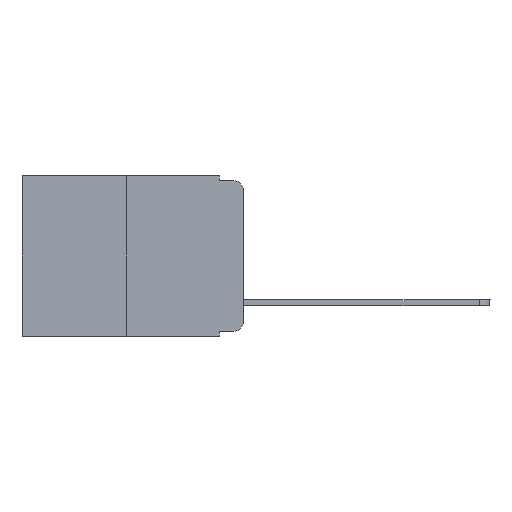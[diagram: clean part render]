
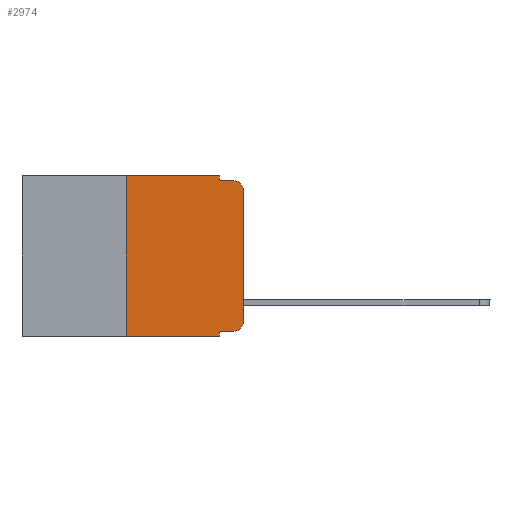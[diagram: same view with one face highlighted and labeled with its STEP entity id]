
A CAD part, left-side view. The second image highlights one B-rep face of the part: STEP entity #2974.
In plain terms, the highlighted planar face has unit normal (-1, 0, 0).
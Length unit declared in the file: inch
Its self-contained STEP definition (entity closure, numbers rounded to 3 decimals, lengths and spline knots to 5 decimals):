
#389 = LINE ( 'NONE', #3741, #22636 ) ;
#976 = CARTESIAN_POINT ( 'NONE',  ( 0., 0.25, 0. ) ) ;
#1397 = DIRECTION ( 'NONE',  ( 0., 0., 1. ) ) ;
#1466 = DIRECTION ( 'NONE',  ( 0., 0., -1. ) ) ;
#1766 = VERTEX_POINT ( 'NONE', #20906 ) ;
#1799 = EDGE_CURVE ( 'NONE', #18498, #20339, #9562, .T. ) ;
#2149 = CARTESIAN_POINT ( 'NONE',  ( 0., 0.25, -0.343 ) ) ;
#2675 = DIRECTION ( 'NONE',  ( 0., -1., 0. ) ) ;
#2742 = CARTESIAN_POINT ( 'NONE',  ( 0., 0.051, -0.333 ) ) ;
#2803 = LINE ( 'NONE', #976, #7537 ) ;
#2889 = DIRECTION ( 'NONE',  ( 0., 0., 1. ) ) ;
#2974 = ADVANCED_FACE ( 'NONE', ( #15620 ), #15904, .F. ) ;
#3198 = EDGE_CURVE ( 'NONE', #24201, #20629, #23777, .T. ) ;
#3352 = LINE ( 'NONE', #2742, #7173 ) ;
#3597 = CARTESIAN_POINT ( 'NONE',  ( 0., 0., -0.313 ) ) ;
#3741 = CARTESIAN_POINT ( 'NONE',  ( 0., 0.051, -0.01 ) ) ;
#4355 = ORIENTED_EDGE ( 'NONE', *, *, #20521, .T. ) ;
#4541 = DIRECTION ( 'NONE',  ( 0., -1., 0. ) ) ;
#4704 = CARTESIAN_POINT ( 'NONE',  ( 0., 0.473, 0. ) ) ;
#4723 = EDGE_CURVE ( 'NONE', #20629, #5110, #20516, .T. ) ;
#5110 = VERTEX_POINT ( 'NONE', #7577 ) ;
#5482 = CARTESIAN_POINT ( 'NONE',  ( 0., 0.051, 0. ) ) ;
#5910 = DIRECTION ( 'NONE',  ( 0., -1., 0. ) ) ;
#6324 = CIRCLE ( 'NONE', #9979, 0.02 ) ;
#6685 = VECTOR ( 'NONE', #2675, 39.37008 ) ;
#7173 = VECTOR ( 'NONE', #4541, 39.37008 ) ;
#7537 = VECTOR ( 'NONE', #2889, 39.37008 ) ;
#7577 = CARTESIAN_POINT ( 'NONE',  ( 0., 0.02, -0.01 ) ) ;
#7585 = VERTEX_POINT ( 'NONE', #2149 ) ;
#7666 = VERTEX_POINT ( 'NONE', #21299 ) ;
#8234 = EDGE_CURVE ( 'NONE', #7585, #7666, #18344, .T. ) ;
#8530 = ORIENTED_EDGE ( 'NONE', *, *, #14546, .F. ) ;
#8667 = EDGE_CURVE ( 'NONE', #7585, #14460, #2803, .T. ) ;
#8802 = AXIS2_PLACEMENT_3D ( 'NONE', #18492, #12857, #1466 ) ;
#9562 = LINE ( 'NONE', #9573, #13900 ) ;
#9573 = CARTESIAN_POINT ( 'NONE',  ( 0., 0.051, 0. ) ) ;
#9606 = ORIENTED_EDGE ( 'NONE', *, *, #1799, .F. ) ;
#9736 = EDGE_CURVE ( 'NONE', #14381, #1766, #3352, .T. ) ;
#9851 = ORIENTED_EDGE ( 'NONE', *, *, #4723, .T. ) ;
#9979 = AXIS2_PLACEMENT_3D ( 'NONE', #14351, #10777, #10848 ) ;
#10173 = EDGE_CURVE ( 'NONE', #14381, #7666, #13553, .T. ) ;
#10641 = VECTOR ( 'NONE', #15260, 39.37008 ) ;
#10777 = DIRECTION ( 'NONE',  ( -1., 0., 0. ) ) ;
#10848 = DIRECTION ( 'NONE',  ( 0., 0., -1. ) ) ;
#11350 = ORIENTED_EDGE ( 'NONE', *, *, #17610, .F. ) ;
#11405 = DIRECTION ( 'NONE',  ( 0., 0., -1. ) ) ;
#12857 = DIRECTION ( 'NONE',  ( -1., 0., 0. ) ) ;
#13503 = EDGE_LOOP ( 'NONE', ( #19435, #9851, #8530, #9606, #11350, #23774, #15756, #16168, #20998, #4355 ) ) ;
#13553 = LINE ( 'NONE', #5482, #10641 ) ;
#13656 = CARTESIAN_POINT ( 'NONE',  ( 0., 0.473, -0.343 ) ) ;
#13900 = VECTOR ( 'NONE', #11405, 39.37008 ) ;
#14351 = CARTESIAN_POINT ( 'NONE',  ( 0., 0.02, -0.313 ) ) ;
#14381 = VERTEX_POINT ( 'NONE', #22117 ) ;
#14460 = VERTEX_POINT ( 'NONE', #14512 ) ;
#14512 = CARTESIAN_POINT ( 'NONE',  ( 0., 0.25, 0. ) ) ;
#14543 = VECTOR ( 'NONE', #19277, 39.37008 ) ;
#14546 = EDGE_CURVE ( 'NONE', #20339, #5110, #389, .T. ) ;
#14588 = LINE ( 'NONE', #17785, #6685 ) ;
#15076 = CARTESIAN_POINT ( 'NONE',  ( 0., 0., -0.03 ) ) ;
#15260 = DIRECTION ( 'NONE',  ( 0., 0., -1. ) ) ;
#15597 = VECTOR ( 'NONE', #1397, 39.37008 ) ;
#15620 = FACE_OUTER_BOUND ( 'NONE', #13503, .T. ) ;
#15756 = ORIENTED_EDGE ( 'NONE', *, *, #8234, .T. ) ;
#15898 = CARTESIAN_POINT ( 'NONE',  ( 0., 0.051, -0.01 ) ) ;
#15904 = PLANE ( 'NONE',  #22057 ) ;
#16168 = ORIENTED_EDGE ( 'NONE', *, *, #10173, .F. ) ;
#16379 = CARTESIAN_POINT ( 'NONE',  ( 0., 0., 0. ) ) ;
#17610 = EDGE_CURVE ( 'NONE', #14460, #18498, #14588, .T. ) ;
#17776 = DIRECTION ( 'NONE',  ( 1., 0., 0. ) ) ;
#17785 = CARTESIAN_POINT ( 'NONE',  ( 0., 0.473, 0. ) ) ;
#18256 = CARTESIAN_POINT ( 'NONE',  ( 0., 0.051, 0. ) ) ;
#18344 = LINE ( 'NONE', #13656, #14543 ) ;
#18492 = CARTESIAN_POINT ( 'NONE',  ( 0., 0.02, -0.03 ) ) ;
#18498 = VERTEX_POINT ( 'NONE', #18256 ) ;
#19277 = DIRECTION ( 'NONE',  ( 0., -1., 0. ) ) ;
#19435 = ORIENTED_EDGE ( 'NONE', *, *, #3198, .T. ) ;
#19662 = DIRECTION ( 'NONE',  ( 0., 0., -1. ) ) ;
#20339 = VERTEX_POINT ( 'NONE', #15898 ) ;
#20516 = CIRCLE ( 'NONE', #8802, 0.02 ) ;
#20521 = EDGE_CURVE ( 'NONE', #1766, #24201, #6324, .T. ) ;
#20629 = VERTEX_POINT ( 'NONE', #15076 ) ;
#20906 = CARTESIAN_POINT ( 'NONE',  ( 0., 0.02, -0.333 ) ) ;
#20998 = ORIENTED_EDGE ( 'NONE', *, *, #9736, .T. ) ;
#21299 = CARTESIAN_POINT ( 'NONE',  ( 0., 0.051, -0.343 ) ) ;
#22057 = AXIS2_PLACEMENT_3D ( 'NONE', #4704, #17776, #19662 ) ;
#22117 = CARTESIAN_POINT ( 'NONE',  ( 0., 0.051, -0.333 ) ) ;
#22636 = VECTOR ( 'NONE', #5910, 39.37008 ) ;
#23774 = ORIENTED_EDGE ( 'NONE', *, *, #8667, .F. ) ;
#23777 = LINE ( 'NONE', #16379, #15597 ) ;
#24201 = VERTEX_POINT ( 'NONE', #3597 ) ;
